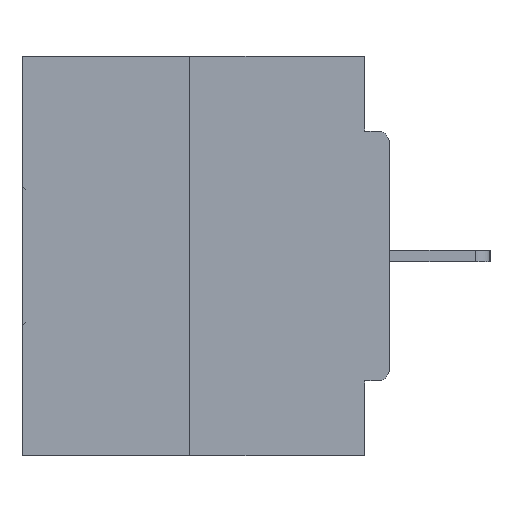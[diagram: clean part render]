
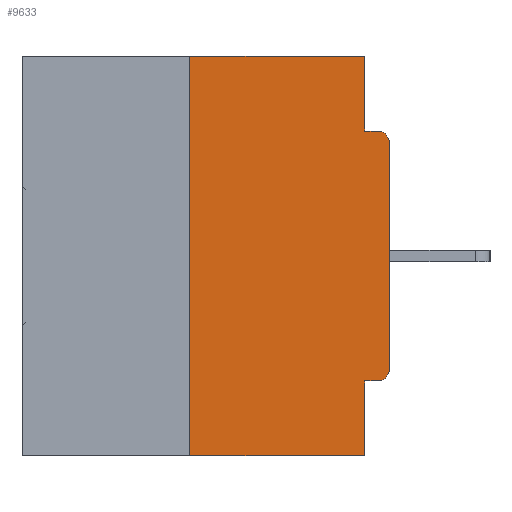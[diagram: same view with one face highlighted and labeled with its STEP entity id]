
A CAD part, left-side view. The second image highlights one B-rep face of the part: STEP entity #9633.
In plain terms, the highlighted planar face has unit normal (-1, 0, 0).
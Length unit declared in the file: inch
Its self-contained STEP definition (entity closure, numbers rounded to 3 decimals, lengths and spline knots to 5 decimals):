
#35 = DIRECTION ( 'NONE',  ( 0., -1., 0. ) ) ;
#99 = CARTESIAN_POINT ( 'NONE',  ( 0., 0.25, -0.5 ) ) ;
#152 = FACE_OUTER_BOUND ( 'NONE', #19459, .T. ) ;
#823 = DIRECTION ( 'NONE',  ( 1., 0., 0. ) ) ;
#948 = EDGE_CURVE ( 'NONE', #15451, #11887, #26510, .T. ) ;
#1569 = DIRECTION ( 'NONE',  ( 0., 0., 1. ) ) ;
#1839 = ORIENTED_EDGE ( 'NONE', *, *, #15496, .F. ) ;
#2285 = VERTEX_POINT ( 'NONE', #7383 ) ;
#2730 = LINE ( 'NONE', #8555, #16181 ) ;
#2819 = EDGE_CURVE ( 'NONE', #22484, #36342, #9661, .T. ) ;
#3613 = DIRECTION ( 'NONE',  ( 0., 0., -1. ) ) ;
#3656 = VERTEX_POINT ( 'NONE', #10656 ) ;
#4985 = DIRECTION ( 'NONE',  ( 0., 0., -1. ) ) ;
#5222 = CARTESIAN_POINT ( 'NONE',  ( 0., 0.031, 0. ) ) ;
#6792 = CARTESIAN_POINT ( 'NONE',  ( 0., 0.46, 0. ) ) ;
#6917 = PLANE ( 'NONE',  #13716 ) ;
#7383 = CARTESIAN_POINT ( 'NONE',  ( 0., 0., -0.3915 ) ) ;
#7428 = VECTOR ( 'NONE', #1569, 39.37008 ) ;
#7569 = CARTESIAN_POINT ( 'NONE',  ( 0., 0.46, 0. ) ) ;
#8043 = EDGE_CURVE ( 'NONE', #22084, #36239, #35122, .T. ) ;
#8555 = CARTESIAN_POINT ( 'NONE',  ( 0., 0., -0.4065 ) ) ;
#8964 = ORIENTED_EDGE ( 'NONE', *, *, #18563, .T. ) ;
#9007 = CARTESIAN_POINT ( 'NONE',  ( 0., 0., -0.1085 ) ) ;
#9633 = ADVANCED_FACE ( 'NONE', ( #152 ), #6917, .F. ) ;
#9661 = LINE ( 'NONE', #33201, #18128 ) ;
#10305 = CARTESIAN_POINT ( 'NONE',  ( 0., 0.25, 0. ) ) ;
#10432 = VECTOR ( 'NONE', #4985, 39.37008 ) ;
#10656 = CARTESIAN_POINT ( 'NONE',  ( 0., 0.015, -0.0935 ) ) ;
#10698 = LINE ( 'NONE', #31648, #32593 ) ;
#11436 = VECTOR ( 'NONE', #36939, 39.37008 ) ;
#11472 = CARTESIAN_POINT ( 'NONE',  ( 0., 0.031, -0.5 ) ) ;
#11887 = VERTEX_POINT ( 'NONE', #11472 ) ;
#13029 = CARTESIAN_POINT ( 'NONE',  ( 0., 0.031, -0.4065 ) ) ;
#13716 = AXIS2_PLACEMENT_3D ( 'NONE', #6792, #823, #3613 ) ;
#14514 = DIRECTION ( 'NONE',  ( 0., 1., 0. ) ) ;
#14914 = CARTESIAN_POINT ( 'NONE',  ( 0., 0.031, -0.0935 ) ) ;
#15004 = ORIENTED_EDGE ( 'NONE', *, *, #31117, .F. ) ;
#15260 = VECTOR ( 'NONE', #35, 39.37008 ) ;
#15451 = VERTEX_POINT ( 'NONE', #13029 ) ;
#15496 = EDGE_CURVE ( 'NONE', #36239, #22484, #30546, .T. ) ;
#15749 = CARTESIAN_POINT ( 'NONE',  ( 0., 0., 0. ) ) ;
#16181 = VECTOR ( 'NONE', #14514, 39.37008 ) ;
#16509 = ORIENTED_EDGE ( 'NONE', *, *, #948, .F. ) ;
#18128 = VECTOR ( 'NONE', #33688, 39.37008 ) ;
#18563 = EDGE_CURVE ( 'NONE', #28855, #3656, #34592, .T. ) ;
#18934 = AXIS2_PLACEMENT_3D ( 'NONE', #34366, #36995, #31243 ) ;
#19459 = EDGE_LOOP ( 'NONE', ( #1839, #20302, #33464, #16509, #29350, #36882, #25388, #8964, #15004, #20223 ) ) ;
#19573 = CIRCLE ( 'NONE', #31705, 0.015 ) ;
#20223 = ORIENTED_EDGE ( 'NONE', *, *, #2819, .F. ) ;
#20302 = ORIENTED_EDGE ( 'NONE', *, *, #8043, .F. ) ;
#22084 = VERTEX_POINT ( 'NONE', #99 ) ;
#22127 = CARTESIAN_POINT ( 'NONE',  ( 0., 0.031, -0.5 ) ) ;
#22484 = VERTEX_POINT ( 'NONE', #5222 ) ;
#22556 = VERTEX_POINT ( 'NONE', #34087 ) ;
#22871 = EDGE_CURVE ( 'NONE', #22084, #11887, #10698, .T. ) ;
#22974 = VECTOR ( 'NONE', #33149, 39.37008 ) ;
#25388 = ORIENTED_EDGE ( 'NONE', *, *, #26285, .T. ) ;
#26285 = EDGE_CURVE ( 'NONE', #2285, #28855, #27961, .T. ) ;
#26510 = LINE ( 'NONE', #22127, #10432 ) ;
#27941 = DIRECTION ( 'NONE',  ( -1., 0., 0. ) ) ;
#27961 = LINE ( 'NONE', #15749, #7428 ) ;
#28855 = VERTEX_POINT ( 'NONE', #9007 ) ;
#29350 = ORIENTED_EDGE ( 'NONE', *, *, #29800, .F. ) ;
#29800 = EDGE_CURVE ( 'NONE', #22556, #15451, #2730, .T. ) ;
#30546 = LINE ( 'NONE', #7569, #22974 ) ;
#30914 = LINE ( 'NONE', #36980, #15260 ) ;
#31066 = CARTESIAN_POINT ( 'NONE',  ( 0., 0.25, 0. ) ) ;
#31117 = EDGE_CURVE ( 'NONE', #36342, #3656, #30914, .T. ) ;
#31243 = DIRECTION ( 'NONE',  ( 0., 0., -1. ) ) ;
#31648 = CARTESIAN_POINT ( 'NONE',  ( 0., 0.46, -0.5 ) ) ;
#31705 = AXIS2_PLACEMENT_3D ( 'NONE', #33566, #27941, #33691 ) ;
#32593 = VECTOR ( 'NONE', #34394, 39.37008 ) ;
#32596 = EDGE_CURVE ( 'NONE', #22556, #2285, #19573, .T. ) ;
#33149 = DIRECTION ( 'NONE',  ( 0., -1., 0. ) ) ;
#33201 = CARTESIAN_POINT ( 'NONE',  ( 0., 0.031, 0. ) ) ;
#33464 = ORIENTED_EDGE ( 'NONE', *, *, #22871, .T. ) ;
#33566 = CARTESIAN_POINT ( 'NONE',  ( 0., 0.015, -0.3915 ) ) ;
#33688 = DIRECTION ( 'NONE',  ( 0., 0., -1. ) ) ;
#33691 = DIRECTION ( 'NONE',  ( 0., 0., -1. ) ) ;
#34087 = CARTESIAN_POINT ( 'NONE',  ( 0., 0.015, -0.4065 ) ) ;
#34366 = CARTESIAN_POINT ( 'NONE',  ( 0., 0.015, -0.1085 ) ) ;
#34394 = DIRECTION ( 'NONE',  ( 0., -1., 0. ) ) ;
#34592 = CIRCLE ( 'NONE', #18934, 0.015 ) ;
#35122 = LINE ( 'NONE', #31066, #11436 ) ;
#36239 = VERTEX_POINT ( 'NONE', #10305 ) ;
#36342 = VERTEX_POINT ( 'NONE', #14914 ) ;
#36882 = ORIENTED_EDGE ( 'NONE', *, *, #32596, .T. ) ;
#36939 = DIRECTION ( 'NONE',  ( 0., 0., 1. ) ) ;
#36980 = CARTESIAN_POINT ( 'NONE',  ( 0., 0., -0.0935 ) ) ;
#36995 = DIRECTION ( 'NONE',  ( -1., 0., 0. ) ) ;
